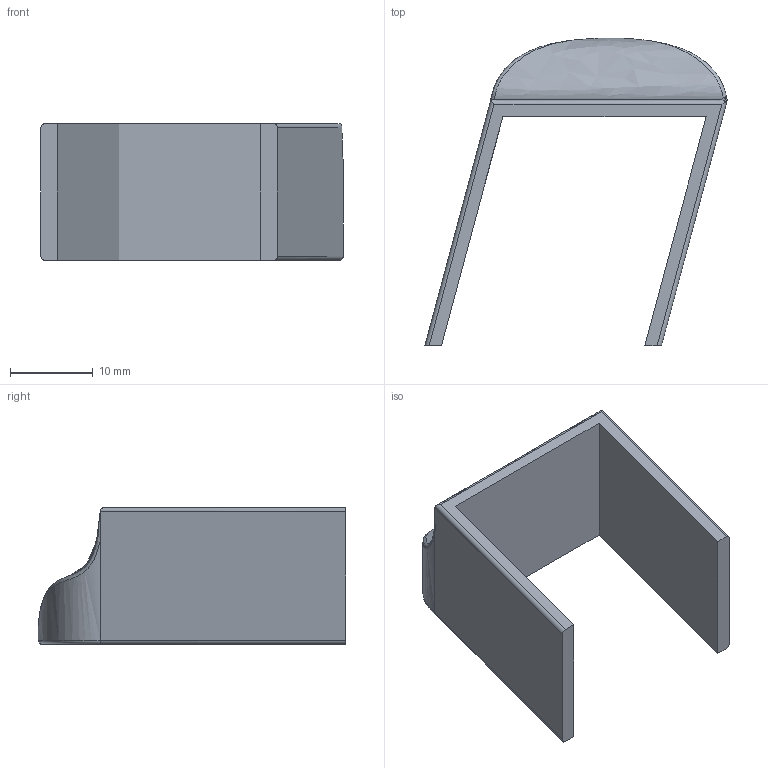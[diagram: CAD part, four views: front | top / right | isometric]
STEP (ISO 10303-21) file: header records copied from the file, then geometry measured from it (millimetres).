
FILE_DESCRIPTION (( 'STEP AP214' ), '1' );
FILE_NAME ('follower.STEP', '2013-06-02T20:16:20', ( '' ), ( '' ), 'SwSTEP 2.0', 'SolidWorks 2013', '' );
FILE_SCHEMA (( 'AUTOMOTIVE_DESIGN' ));
Length unit declared in the file: millimetre
Products named in the file (1): follower
Bounding box: 36.42 x 37.09 x 16.5 mm (x, y, z)
Volume: 4268.7 mm3; surface area: 3498.4 mm2
Topology: 1 solids, 1 shells, 25 faces, 60 edges, 37 vertices
Faces by surface type: plane 10, bspline 6, cylinder 5, sphere 4
Entity records: 1441 total; most frequent: CARTESIAN_POINT 886, ORIENTED_EDGE 120, DIRECTION 90, EDGE_CURVE 60, VERTEX_POINT 37, AXIS2_PLACEMENT_3D 31, VECTOR 28, LINE 28
